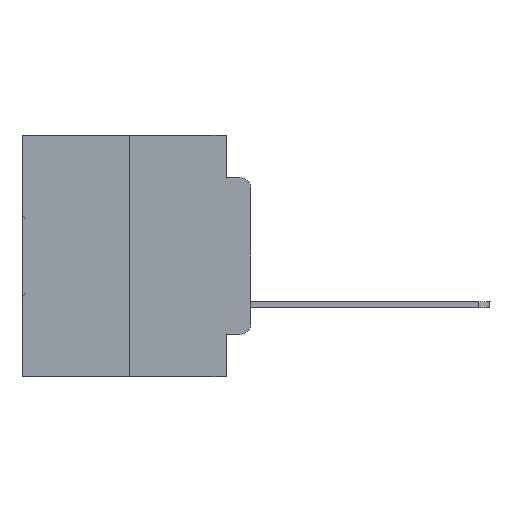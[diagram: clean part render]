
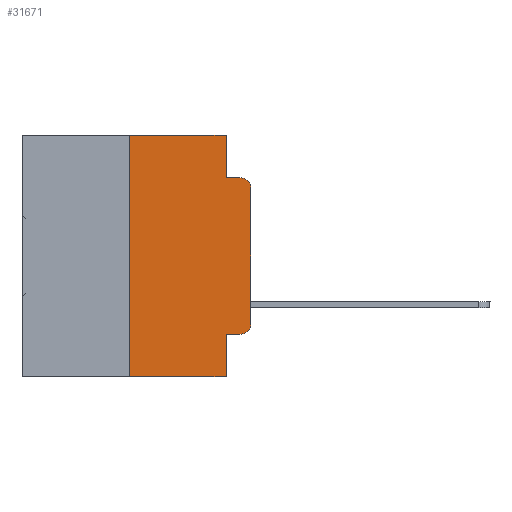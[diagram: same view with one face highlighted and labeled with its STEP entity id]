
A CAD part, left-side view. The second image highlights one B-rep face of the part: STEP entity #31671.
In plain terms, the highlighted planar face has unit normal (-1, 0, 0).
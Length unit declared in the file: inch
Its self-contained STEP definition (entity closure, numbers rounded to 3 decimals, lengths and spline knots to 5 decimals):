
#330 = DIRECTION ( 'NONE',  ( 0., 0., -1. ) ) ;
#388 = DIRECTION ( 'NONE',  ( 0., -1., 0. ) ) ;
#498 = LINE ( 'NONE', #19606, #20898 ) ;
#1266 = DIRECTION ( 'NONE',  ( 0., 0., -1. ) ) ;
#1576 = ORIENTED_EDGE ( 'NONE', *, *, #26367, .F. ) ;
#1891 = EDGE_CURVE ( 'NONE', #14686, #28521, #498, .T. ) ;
#2098 = LINE ( 'NONE', #30162, #24920 ) ;
#2795 = DIRECTION ( 'NONE',  ( 1., 0., 0. ) ) ;
#2796 = EDGE_CURVE ( 'NONE', #30212, #14686, #28131, .T. ) ;
#3109 = CARTESIAN_POINT ( 'NONE',  ( 0., 0.473, -0.5 ) ) ;
#4029 = VERTEX_POINT ( 'NONE', #8714 ) ;
#5560 = CARTESIAN_POINT ( 'NONE',  ( 0., 0.25, -0.5 ) ) ;
#6026 = ORIENTED_EDGE ( 'NONE', *, *, #16585, .T. ) ;
#6692 = AXIS2_PLACEMENT_3D ( 'NONE', #14890, #9853, #25528 ) ;
#6869 = CIRCLE ( 'NONE', #6692, 0.02 ) ;
#7406 = CARTESIAN_POINT ( 'NONE',  ( 0., 0.25, 0. ) ) ;
#7823 = CARTESIAN_POINT ( 'NONE',  ( 0., 0.473, 0. ) ) ;
#8437 = CARTESIAN_POINT ( 'NONE',  ( 0., 0.051, 0. ) ) ;
#8714 = CARTESIAN_POINT ( 'NONE',  ( 0., 0.051, -0.5 ) ) ;
#8906 = ORIENTED_EDGE ( 'NONE', *, *, #31687, .F. ) ;
#9825 = AXIS2_PLACEMENT_3D ( 'NONE', #7823, #2795, #18298 ) ;
#9853 = DIRECTION ( 'NONE',  ( -1., 0., 0. ) ) ;
#10268 = LINE ( 'NONE', #23518, #13562 ) ;
#10335 = EDGE_CURVE ( 'NONE', #25050, #4029, #18568, .T. ) ;
#10890 = LINE ( 'NONE', #7406, #19439 ) ;
#11823 = CARTESIAN_POINT ( 'NONE',  ( 0., 0., -0.3915 ) ) ;
#12121 = VERTEX_POINT ( 'NONE', #26760 ) ;
#12152 = DIRECTION ( 'NONE',  ( -1., 0., 0. ) ) ;
#12830 = ORIENTED_EDGE ( 'NONE', *, *, #31992, .T. ) ;
#13299 = VECTOR ( 'NONE', #13970, 39.37008 ) ;
#13562 = VECTOR ( 'NONE', #388, 39.37008 ) ;
#13970 = DIRECTION ( 'NONE',  ( 0., -1., 0. ) ) ;
#14686 = VERTEX_POINT ( 'NONE', #27060 ) ;
#14890 = CARTESIAN_POINT ( 'NONE',  ( 0., 0.02, -0.3915 ) ) ;
#15806 = VERTEX_POINT ( 'NONE', #30067 ) ;
#16022 = FACE_OUTER_BOUND ( 'NONE', #18417, .T. ) ;
#16192 = DIRECTION ( 'NONE',  ( 0., -1., 0. ) ) ;
#16306 = VECTOR ( 'NONE', #16192, 39.37008 ) ;
#16585 = EDGE_CURVE ( 'NONE', #23506, #25918, #6869, .T. ) ;
#16913 = CARTESIAN_POINT ( 'NONE',  ( 0., 0.051, 0. ) ) ;
#17221 = DIRECTION ( 'NONE',  ( 0., -1., 0. ) ) ;
#17233 = EDGE_CURVE ( 'NONE', #25050, #15806, #10890, .T. ) ;
#18298 = DIRECTION ( 'NONE',  ( 0., 0., -1. ) ) ;
#18417 = EDGE_LOOP ( 'NONE', ( #21719, #12830, #19360, #26498, #8906, #26747, #21872, #1576, #21764, #6026 ) ) ;
#18568 = LINE ( 'NONE', #3109, #13299 ) ;
#19360 = ORIENTED_EDGE ( 'NONE', *, *, #1891, .F. ) ;
#19438 = VERTEX_POINT ( 'NONE', #31017 ) ;
#19439 = VECTOR ( 'NONE', #28216, 39.37008 ) ;
#19606 = CARTESIAN_POINT ( 'NONE',  ( 0., 0.051, -0.0885 ) ) ;
#20522 = EDGE_CURVE ( 'NONE', #25918, #12121, #2098, .T. ) ;
#20771 = LINE ( 'NONE', #21320, #16306 ) ;
#20824 = PLANE ( 'NONE',  #9825 ) ;
#20898 = VECTOR ( 'NONE', #17221, 39.37008 ) ;
#21320 = CARTESIAN_POINT ( 'NONE',  ( 0., 0.051, -0.4115 ) ) ;
#21719 = ORIENTED_EDGE ( 'NONE', *, *, #20522, .T. ) ;
#21764 = ORIENTED_EDGE ( 'NONE', *, *, #32988, .T. ) ;
#21851 = VECTOR ( 'NONE', #1266, 39.37008 ) ;
#21872 = ORIENTED_EDGE ( 'NONE', *, *, #10335, .T. ) ;
#22611 = CARTESIAN_POINT ( 'NONE',  ( 0., 0.02, -0.4115 ) ) ;
#23506 = VERTEX_POINT ( 'NONE', #22611 ) ;
#23518 = CARTESIAN_POINT ( 'NONE',  ( 0., 0.473, 0. ) ) ;
#24495 = VECTOR ( 'NONE', #330, 39.37008 ) ;
#24558 = DIRECTION ( 'NONE',  ( 0., 0., 1. ) ) ;
#24920 = VECTOR ( 'NONE', #24558, 39.37008 ) ;
#25050 = VERTEX_POINT ( 'NONE', #5560 ) ;
#25528 = DIRECTION ( 'NONE',  ( 0., 0., -1. ) ) ;
#25699 = CIRCLE ( 'NONE', #31662, 0.02 ) ;
#25748 = CARTESIAN_POINT ( 'NONE',  ( 0., 0.051, 0. ) ) ;
#25918 = VERTEX_POINT ( 'NONE', #11823 ) ;
#26367 = EDGE_CURVE ( 'NONE', #19438, #4029, #28755, .T. ) ;
#26498 = ORIENTED_EDGE ( 'NONE', *, *, #2796, .F. ) ;
#26747 = ORIENTED_EDGE ( 'NONE', *, *, #17233, .F. ) ;
#26760 = CARTESIAN_POINT ( 'NONE',  ( 0., 0., -0.1085 ) ) ;
#27060 = CARTESIAN_POINT ( 'NONE',  ( 0., 0.051, -0.0885 ) ) ;
#27600 = DIRECTION ( 'NONE',  ( 0., 0., -1. ) ) ;
#28131 = LINE ( 'NONE', #8437, #24495 ) ;
#28216 = DIRECTION ( 'NONE',  ( 0., 0., 1. ) ) ;
#28521 = VERTEX_POINT ( 'NONE', #31186 ) ;
#28755 = LINE ( 'NONE', #16913, #21851 ) ;
#30067 = CARTESIAN_POINT ( 'NONE',  ( 0., 0.25, 0. ) ) ;
#30162 = CARTESIAN_POINT ( 'NONE',  ( 0., 0., 0. ) ) ;
#30212 = VERTEX_POINT ( 'NONE', #25748 ) ;
#30588 = CARTESIAN_POINT ( 'NONE',  ( 0., 0.02, -0.1085 ) ) ;
#31017 = CARTESIAN_POINT ( 'NONE',  ( 0., 0.051, -0.4115 ) ) ;
#31186 = CARTESIAN_POINT ( 'NONE',  ( 0., 0.02, -0.0885 ) ) ;
#31662 = AXIS2_PLACEMENT_3D ( 'NONE', #30588, #12152, #27600 ) ;
#31671 = ADVANCED_FACE ( 'NONE', ( #16022 ), #20824, .F. ) ;
#31687 = EDGE_CURVE ( 'NONE', #15806, #30212, #10268, .T. ) ;
#31992 = EDGE_CURVE ( 'NONE', #12121, #28521, #25699, .T. ) ;
#32988 = EDGE_CURVE ( 'NONE', #19438, #23506, #20771, .T. ) ;
